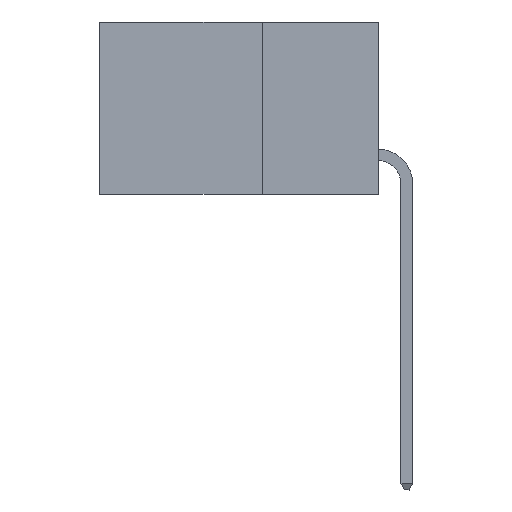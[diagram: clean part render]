
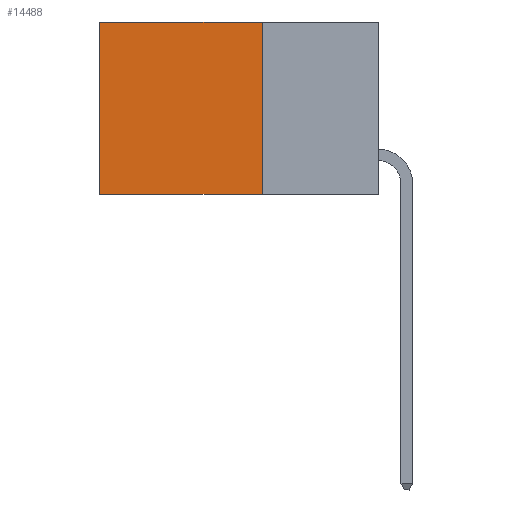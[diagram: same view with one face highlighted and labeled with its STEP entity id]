
A CAD part, left-side view. The second image highlights one B-rep face of the part: STEP entity #14488.
In plain terms, the highlighted planar face has unit normal (-1, 0, 0).
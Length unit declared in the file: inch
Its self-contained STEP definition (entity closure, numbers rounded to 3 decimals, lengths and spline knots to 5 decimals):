
#200 = EDGE_CURVE ( 'NONE', #19156, #17142, #12385, .T. ) ;
#276 = ORIENTED_EDGE ( 'NONE', *, *, #7180, .T. ) ;
#3008 = CARTESIAN_POINT ( 'NONE',  ( 0.2615, 0.25, -0.37 ) ) ;
#6043 = VERTEX_POINT ( 'NONE', #21432 ) ;
#6175 = VERTEX_POINT ( 'NONE', #12157 ) ;
#6617 = LINE ( 'NONE', #14489, #12306 ) ;
#7034 = LINE ( 'NONE', #14901, #9576 ) ;
#7180 = EDGE_CURVE ( 'NONE', #6175, #6043, #7034, .T. ) ;
#7400 = DIRECTION ( 'NONE',  ( 1., 0., 0. ) ) ;
#9462 = FACE_OUTER_BOUND ( 'NONE', #11258, .T. ) ;
#9576 = VECTOR ( 'NONE', #9951, 39.37008 ) ;
#9951 = DIRECTION ( 'NONE',  ( 0., 1., 0. ) ) ;
#10750 = DIRECTION ( 'NONE',  ( 0., 0., -1. ) ) ;
#11149 = ORIENTED_EDGE ( 'NONE', *, *, #200, .F. ) ;
#11258 = EDGE_LOOP ( 'NONE', ( #20058, #11149, #15935, #276 ) ) ;
#11510 = EDGE_CURVE ( 'NONE', #6043, #17142, #6617, .T. ) ;
#12157 = CARTESIAN_POINT ( 'NONE',  ( 0.2615, 0.25, 0. ) ) ;
#12271 = DIRECTION ( 'NONE',  ( 0., 0., -1. ) ) ;
#12306 = VECTOR ( 'NONE', #10750, 39.37008 ) ;
#12385 = LINE ( 'NONE', #16255, #15170 ) ;
#12644 = DIRECTION ( 'NONE',  ( 0., 1., 0. ) ) ;
#13341 = PLANE ( 'NONE',  #16627 ) ;
#14062 = CARTESIAN_POINT ( 'NONE',  ( 0.2615, 0.25, -0.37 ) ) ;
#14488 = ADVANCED_FACE ( 'NONE', ( #9462 ), #13341, .F. ) ;
#14489 = CARTESIAN_POINT ( 'NONE',  ( 0.2615, 0.6, -0.37 ) ) ;
#14901 = CARTESIAN_POINT ( 'NONE',  ( 0.2615, 0.25, 0. ) ) ;
#15170 = VECTOR ( 'NONE', #12644, 39.37008 ) ;
#15190 = CARTESIAN_POINT ( 'NONE',  ( 0.2615, 0.25, -0.37 ) ) ;
#15324 = EDGE_CURVE ( 'NONE', #6175, #19156, #16389, .T. ) ;
#15935 = ORIENTED_EDGE ( 'NONE', *, *, #15324, .F. ) ;
#16255 = CARTESIAN_POINT ( 'NONE',  ( 0.2615, 0.25, -0.37 ) ) ;
#16389 = LINE ( 'NONE', #14062, #22403 ) ;
#16627 = AXIS2_PLACEMENT_3D ( 'NONE', #3008, #7400, #21213 ) ;
#17142 = VERTEX_POINT ( 'NONE', #19421 ) ;
#19156 = VERTEX_POINT ( 'NONE', #15190 ) ;
#19421 = CARTESIAN_POINT ( 'NONE',  ( 0.2615, 0.6, -0.37 ) ) ;
#20058 = ORIENTED_EDGE ( 'NONE', *, *, #11510, .T. ) ;
#21213 = DIRECTION ( 'NONE',  ( 0., 0., -1. ) ) ;
#21432 = CARTESIAN_POINT ( 'NONE',  ( 0.2615, 0.6, 0. ) ) ;
#22403 = VECTOR ( 'NONE', #12271, 39.37008 ) ;
